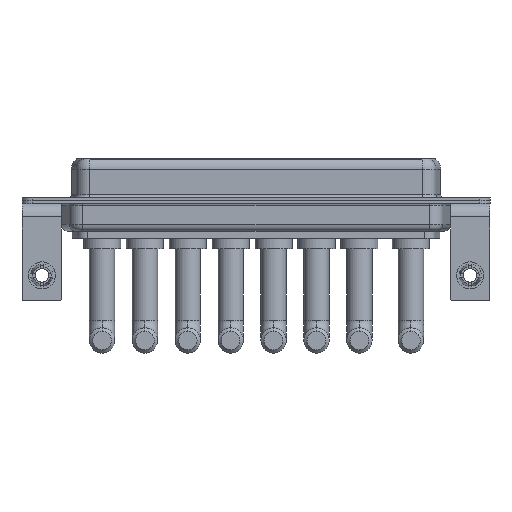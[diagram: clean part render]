
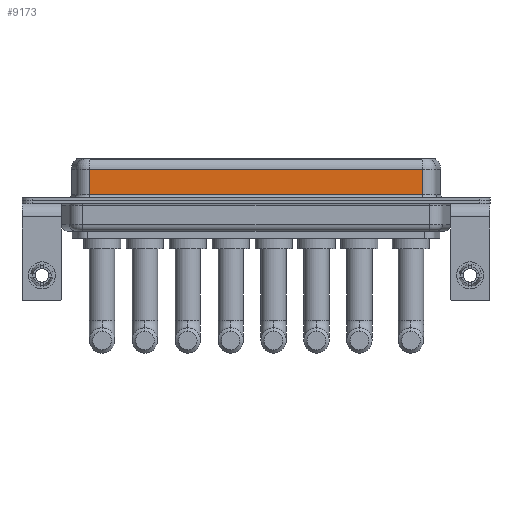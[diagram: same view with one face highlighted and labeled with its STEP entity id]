
A CAD part, front view. The second image highlights one B-rep face of the part: STEP entity #9173.
In plain terms, the highlighted planar face has unit normal (0, -1, 0).
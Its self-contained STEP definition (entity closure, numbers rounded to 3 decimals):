
#238 = EDGE_LOOP ( 'NONE', ( #7660, #1151, #5508, #1171 ) ) ;
#1140 = CARTESIAN_POINT ( 'NONE',  ( 56.462, -3.95, 0.9 ) ) ;
#1151 = ORIENTED_EDGE ( 'NONE', *, *, #7166, .T. ) ;
#1171 = ORIENTED_EDGE ( 'NONE', *, *, #3526, .T. ) ;
#2031 = LINE ( 'NONE', #10448, #5196 ) ;
#2180 = LINE ( 'NONE', #15520, #11820 ) ;
#2786 = VERTEX_POINT ( 'NONE', #6941 ) ;
#3198 = DIRECTION ( 'NONE',  ( 0., 0., 1. ) ) ;
#3526 = EDGE_CURVE ( 'NONE', #10569, #11443, #11149, .T. ) ;
#4393 = CARTESIAN_POINT ( 'NONE',  ( 56.462, -3.95, 6.4 ) ) ;
#4490 = DIRECTION ( 'NONE',  ( -1., 0., 0. ) ) ;
#4594 = DIRECTION ( 'NONE',  ( 0., 0., -1. ) ) ;
#4618 = VECTOR ( 'NONE', #4594, 1000. ) ;
#5196 = VECTOR ( 'NONE', #4490, 1000. ) ;
#5319 = CARTESIAN_POINT ( 'NONE',  ( 56.462, -3.95, 0.9 ) ) ;
#5508 = ORIENTED_EDGE ( 'NONE', *, *, #7153, .T. ) ;
#5799 = CARTESIAN_POINT ( 'NONE',  ( 56.462, -3.95, 6.4 ) ) ;
#6941 = CARTESIAN_POINT ( 'NONE',  ( 56.462, -3.95, 4.65 ) ) ;
#7024 = VECTOR ( 'NONE', #7193, 1000. ) ;
#7153 = EDGE_CURVE ( 'NONE', #11109, #10569, #2180, .T. ) ;
#7166 = EDGE_CURVE ( 'NONE', #2786, #11109, #2031, .T. ) ;
#7193 = DIRECTION ( 'NONE',  ( 1., 0., 0. ) ) ;
#7660 = ORIENTED_EDGE ( 'NONE', *, *, #11497, .F. ) ;
#7901 = CARTESIAN_POINT ( 'NONE',  ( 7.038, -3.95, 4.65 ) ) ;
#8357 = LINE ( 'NONE', #5799, #4618 ) ;
#9173 = ADVANCED_FACE ( 'NONE', ( #15283 ), #11796, .F. ) ;
#10099 = AXIS2_PLACEMENT_3D ( 'NONE', #4393, #15362, #3198 ) ;
#10448 = CARTESIAN_POINT ( 'NONE',  ( 56.462, -3.95, 4.65 ) ) ;
#10569 = VERTEX_POINT ( 'NONE', #15228 ) ;
#11109 = VERTEX_POINT ( 'NONE', #7901 ) ;
#11149 = LINE ( 'NONE', #1140, #7024 ) ;
#11443 = VERTEX_POINT ( 'NONE', #5319 ) ;
#11497 = EDGE_CURVE ( 'NONE', #2786, #11443, #8357, .T. ) ;
#11796 = PLANE ( 'NONE',  #10099 ) ;
#11820 = VECTOR ( 'NONE', #11887, 1000. ) ;
#11887 = DIRECTION ( 'NONE',  ( 0., 0., -1. ) ) ;
#15228 = CARTESIAN_POINT ( 'NONE',  ( 7.038, -3.95, 0.9 ) ) ;
#15283 = FACE_OUTER_BOUND ( 'NONE', #238, .T. ) ;
#15362 = DIRECTION ( 'NONE',  ( 0., 1., 0. ) ) ;
#15520 = CARTESIAN_POINT ( 'NONE',  ( 7.038, -3.95, 6.4 ) ) ;
